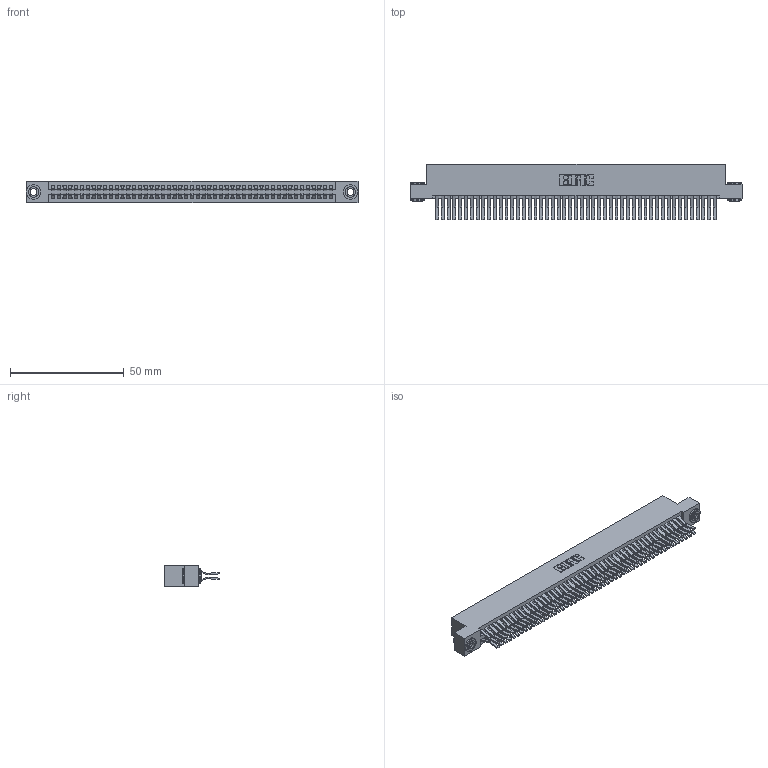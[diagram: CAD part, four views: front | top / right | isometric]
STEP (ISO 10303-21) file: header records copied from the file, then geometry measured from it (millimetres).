
FILE_DESCRIPTION (( 'STEP AP203' ), '1' );
FILE_NAME ('395-098-560-203.STEP', '2018-11-29T23:05:06', ( '' ), ( '' ), 'SwSTEP 2.0', 'SolidWorks 2016', '' );
FILE_SCHEMA (( 'CONFIG_CONTROL_DESIGN' ));
Length unit declared in the file: inch
Products named in the file (4): 345-292-001_560 Tail; 345 Part_Flush Mounting Lugs - 0.156 Dia-TH; 345-250-002_345-250-002-102; 395-098-560-203
Assembly tree (101 placements, depth 2):
  395-098-560-203
    345 Part_Flush Mounting Lugs - 0.156 Dia-TH
    345-292-001_560 Tail  x98
    345-250-002_345-250-002-102  x2
Bounding box: 145.67 x 24.45 x 9.4 mm (x, y, z)
Volume: 14877.2 mm3; surface area: 23983.5 mm2
Topology: 101 solids, 101 shells, 5260 faces, 15607 edges, 10270 vertices
Faces by surface type: plane 3324, cylinder 1928, cone 8
Entity records: 38242 total; most frequent: CARTESIAN_POINT 6379, ORIENTED_EDGE 6306, DIRECTION 5651, EDGE_CURVE 3153, LINE 2797, VECTOR 2797, VERTEX_POINT 2098, AXIS2_PLACEMENT_3D 1427
